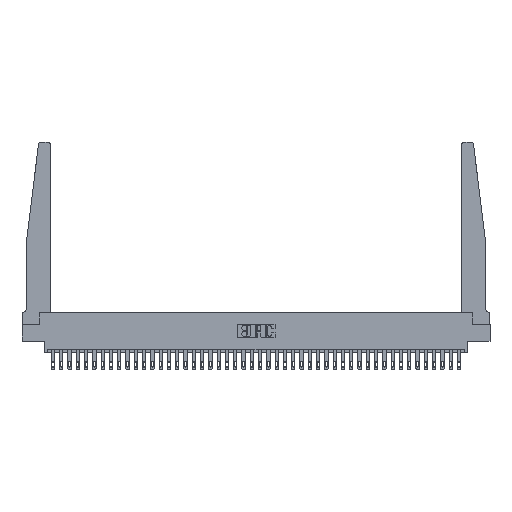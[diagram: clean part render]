
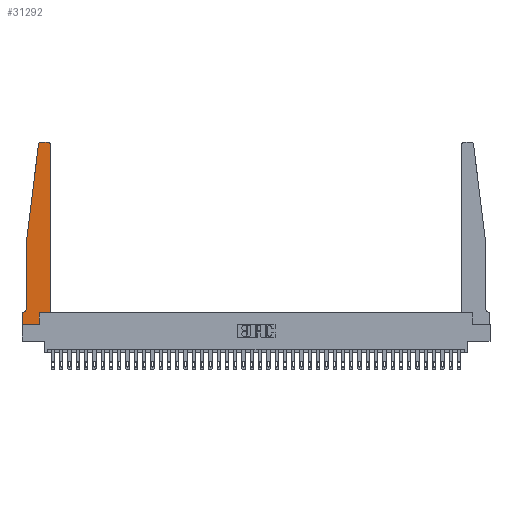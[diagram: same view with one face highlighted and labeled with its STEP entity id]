
A CAD part, top view. The second image highlights one B-rep face of the part: STEP entity #31292.
In plain terms, the highlighted planar face has unit normal (0, 0, 1).
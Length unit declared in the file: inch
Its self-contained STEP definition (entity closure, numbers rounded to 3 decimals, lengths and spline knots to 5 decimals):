
#664 = VERTEX_POINT ( 'NONE', #18329 ) ;
#841 = CARTESIAN_POINT ( 'NONE',  ( 0.27653, 2.75, 0.37 ) ) ;
#866 = EDGE_CURVE ( 'NONE', #28639, #16519, #30469, .T. ) ;
#1304 = EDGE_CURVE ( 'NONE', #4765, #18674, #24430, .T. ) ;
#2855 = EDGE_CURVE ( 'NONE', #16519, #30853, #27185, .T. ) ;
#3380 = ORIENTED_EDGE ( 'NONE', *, *, #25129, .T. ) ;
#4038 = CARTESIAN_POINT ( 'NONE',  ( 0.015, 0.1875, 0.37 ) ) ;
#4137 = EDGE_CURVE ( 'NONE', #35445, #4765, #9280, .T. ) ;
#4404 = LINE ( 'NONE', #4586, #16518 ) ;
#4430 = VERTEX_POINT ( 'NONE', #9082 ) ;
#4586 = CARTESIAN_POINT ( 'NONE',  ( 0.065, 1.25, 0.37 ) ) ;
#4765 = VERTEX_POINT ( 'NONE', #4038 ) ;
#5318 = EDGE_CURVE ( 'NONE', #4430, #16106, #35841, .T. ) ;
#5711 = FACE_OUTER_BOUND ( 'NONE', #7492, .T. ) ;
#5866 = ORIENTED_EDGE ( 'NONE', *, *, #11239, .T. ) ;
#6253 = PLANE ( 'NONE',  #30001 ) ;
#6258 = DIRECTION ( 'NONE',  ( -0.122, -0.992, 0. ) ) ;
#7220 = CARTESIAN_POINT ( 'NONE',  ( 0.425, 0.18, 0.37 ) ) ;
#7233 = CARTESIAN_POINT ( 'NONE',  ( 0.065, 1.25, 0.37 ) ) ;
#7238 = DIRECTION ( 'NONE',  ( 0., 1., 0. ) ) ;
#7492 = EDGE_LOOP ( 'NONE', ( #23851, #24910, #7721, #3380, #14566, #28616, #13613, #36675, #15368, #20819, #5866, #14125 ) ) ;
#7721 = ORIENTED_EDGE ( 'NONE', *, *, #11522, .T. ) ;
#7764 = DIRECTION ( 'NONE',  ( 0., 1., 0. ) ) ;
#7820 = CARTESIAN_POINT ( 'NONE',  ( 0.065, 0.1875, 0.37 ) ) ;
#9082 = CARTESIAN_POINT ( 'NONE',  ( 0.395, 2.75, 0.37 ) ) ;
#9154 = DIRECTION ( 'NONE',  ( 0., -1., 0. ) ) ;
#9239 = LINE ( 'NONE', #26776, #12418 ) ;
#9280 = CIRCLE ( 'NONE', #35497, 0.05 ) ;
#9374 = VECTOR ( 'NONE', #7764, 39.37008 ) ;
#10223 = DIRECTION ( 'NONE',  ( 0., 0., -1. ) ) ;
#10742 = LINE ( 'NONE', #7220, #9374 ) ;
#11239 = EDGE_CURVE ( 'NONE', #18576, #15763, #10742, .T. ) ;
#11522 = EDGE_CURVE ( 'NONE', #664, #15219, #9239, .T. ) ;
#12159 = EDGE_CURVE ( 'NONE', #30853, #18576, #30767, .T. ) ;
#12418 = VECTOR ( 'NONE', #6258, 39.37008 ) ;
#13215 = DIRECTION ( 'NONE',  ( -1., 0., 0. ) ) ;
#13378 = EDGE_CURVE ( 'NONE', #18674, #28639, #17178, .T. ) ;
#13401 = AXIS2_PLACEMENT_3D ( 'NONE', #16283, #36624, #16460 ) ;
#13613 = ORIENTED_EDGE ( 'NONE', *, *, #13378, .T. ) ;
#13650 = DIRECTION ( 'NONE',  ( 1., 0., 0. ) ) ;
#14086 = DIRECTION ( 'NONE',  ( 0., 0., 1. ) ) ;
#14125 = ORIENTED_EDGE ( 'NONE', *, *, #22426, .T. ) ;
#14566 = ORIENTED_EDGE ( 'NONE', *, *, #4137, .T. ) ;
#15219 = VERTEX_POINT ( 'NONE', #7233 ) ;
#15368 = ORIENTED_EDGE ( 'NONE', *, *, #2855, .T. ) ;
#15763 = VERTEX_POINT ( 'NONE', #33651 ) ;
#16106 = VERTEX_POINT ( 'NONE', #841 ) ;
#16283 = CARTESIAN_POINT ( 'NONE',  ( 0.27653, 2.72, 0.37 ) ) ;
#16460 = DIRECTION ( 'NONE',  ( 1., 0., 0. ) ) ;
#16518 = VECTOR ( 'NONE', #21181, 39.37008 ) ;
#16519 = VERTEX_POINT ( 'NONE', #32616 ) ;
#17178 = LINE ( 'NONE', #23496, #19691 ) ;
#17440 = CARTESIAN_POINT ( 'NONE',  ( 0., 0.1875, 0.37 ) ) ;
#18225 = CARTESIAN_POINT ( 'NONE',  ( 0.065, 0.2375, 0.37 ) ) ;
#18329 = CARTESIAN_POINT ( 'NONE',  ( 0.24675, 2.72367, 0.37 ) ) ;
#18576 = VERTEX_POINT ( 'NONE', #24703 ) ;
#18674 = VERTEX_POINT ( 'NONE', #35696 ) ;
#18804 = CARTESIAN_POINT ( 'NONE',  ( 0.015, 0.2375, 0.37 ) ) ;
#19691 = VECTOR ( 'NONE', #9154, 39.37008 ) ;
#19705 = VECTOR ( 'NONE', #24787, 39.37008 ) ;
#20819 = ORIENTED_EDGE ( 'NONE', *, *, #12159, .T. ) ;
#21181 = DIRECTION ( 'NONE',  ( 0., -1., 0. ) ) ;
#21412 = EDGE_CURVE ( 'NONE', #16106, #664, #34880, .T. ) ;
#22426 = EDGE_CURVE ( 'NONE', #15763, #4430, #31180, .T. ) ;
#23379 = CARTESIAN_POINT ( 'NONE',  ( 0.395, 2.72, 0.37 ) ) ;
#23496 = CARTESIAN_POINT ( 'NONE',  ( 0., 0., 0.37 ) ) ;
#23569 = DIRECTION ( 'NONE',  ( 0., 0., 1. ) ) ;
#23851 = ORIENTED_EDGE ( 'NONE', *, *, #5318, .T. ) ;
#24430 = LINE ( 'NONE', #7820, #19705 ) ;
#24604 = DIRECTION ( 'NONE',  ( 1., 0., 0. ) ) ;
#24703 = CARTESIAN_POINT ( 'NONE',  ( 0.425, 0.18, 0.37 ) ) ;
#24787 = DIRECTION ( 'NONE',  ( -1., 0., 0. ) ) ;
#24792 = VECTOR ( 'NONE', #29876, 39.37008 ) ;
#24910 = ORIENTED_EDGE ( 'NONE', *, *, #21412, .T. ) ;
#25129 = EDGE_CURVE ( 'NONE', #15219, #35445, #4404, .T. ) ;
#26776 = CARTESIAN_POINT ( 'NONE',  ( 0.065, 1.25, 0.37 ) ) ;
#27067 = VECTOR ( 'NONE', #7238, 39.37008 ) ;
#27185 = LINE ( 'NONE', #30561, #27067 ) ;
#27434 = CARTESIAN_POINT ( 'NONE',  ( 0.25, 2.75, 0.37 ) ) ;
#28457 = DIRECTION ( 'NONE',  ( 1., 0., 0. ) ) ;
#28616 = ORIENTED_EDGE ( 'NONE', *, *, #1304, .T. ) ;
#28639 = VERTEX_POINT ( 'NONE', #36489 ) ;
#29194 = DIRECTION ( 'NONE',  ( 1., 0., 0. ) ) ;
#29876 = DIRECTION ( 'NONE',  ( -1., 0., 0. ) ) ;
#30001 = AXIS2_PLACEMENT_3D ( 'NONE', #17440, #14086, #28457 ) ;
#30469 = LINE ( 'NONE', #33054, #31004 ) ;
#30561 = CARTESIAN_POINT ( 'NONE',  ( 0.2605, 0.18, 0.37 ) ) ;
#30767 = LINE ( 'NONE', #36556, #31522 ) ;
#30853 = VERTEX_POINT ( 'NONE', #31305 ) ;
#31004 = VECTOR ( 'NONE', #13650, 39.37008 ) ;
#31180 = CIRCLE ( 'NONE', #34762, 0.03 ) ;
#31292 = ADVANCED_FACE ( 'NONE', ( #5711 ), #6253, .T. ) ;
#31305 = CARTESIAN_POINT ( 'NONE',  ( 0.2605, 0.18, 0.37 ) ) ;
#31522 = VECTOR ( 'NONE', #24604, 39.37008 ) ;
#32616 = CARTESIAN_POINT ( 'NONE',  ( 0.2605, 0., 0.37 ) ) ;
#33054 = CARTESIAN_POINT ( 'NONE',  ( 0., 0., 0.37 ) ) ;
#33651 = CARTESIAN_POINT ( 'NONE',  ( 0.425, 2.72, 0.37 ) ) ;
#34762 = AXIS2_PLACEMENT_3D ( 'NONE', #23379, #23569, #29194 ) ;
#34880 = CIRCLE ( 'NONE', #13401, 0.03 ) ;
#35445 = VERTEX_POINT ( 'NONE', #18225 ) ;
#35497 = AXIS2_PLACEMENT_3D ( 'NONE', #18804, #10223, #13215 ) ;
#35696 = CARTESIAN_POINT ( 'NONE',  ( 0., 0.1875, 0.37 ) ) ;
#35841 = LINE ( 'NONE', #27434, #24792 ) ;
#36489 = CARTESIAN_POINT ( 'NONE',  ( 0., 0., 0.37 ) ) ;
#36556 = CARTESIAN_POINT ( 'NONE',  ( 0.425, 0.18, 0.37 ) ) ;
#36624 = DIRECTION ( 'NONE',  ( 0., 0., 1. ) ) ;
#36675 = ORIENTED_EDGE ( 'NONE', *, *, #866, .T. ) ;
